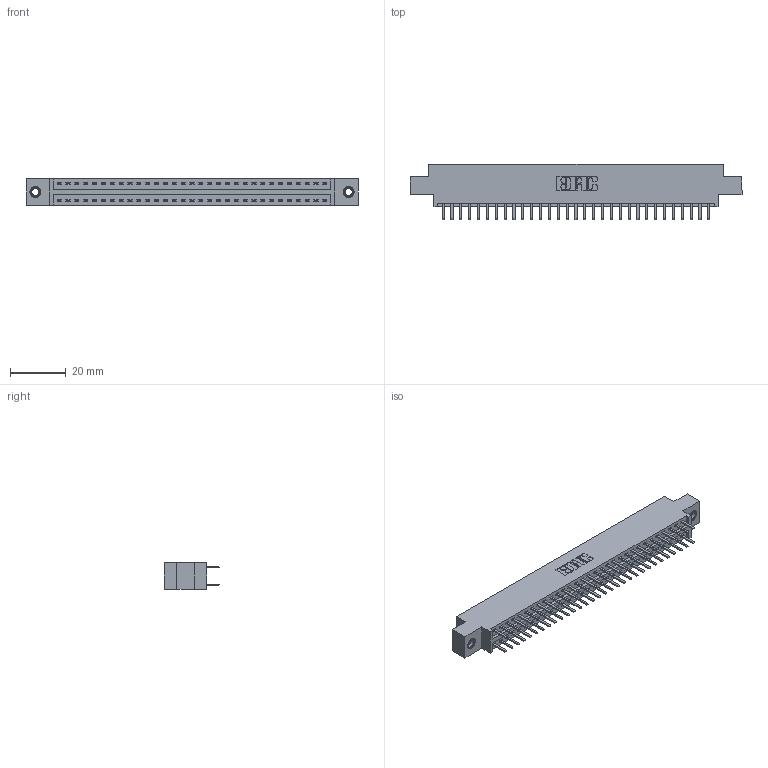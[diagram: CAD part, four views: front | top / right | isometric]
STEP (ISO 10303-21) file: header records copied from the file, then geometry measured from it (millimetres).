
FILE_DESCRIPTION (( 'STEP AP203' ), '1' );
FILE_NAME ('396-062-520-807.STEP', '2019-11-02T09:13:12', ( '' ), ( '' ), 'SwSTEP 2.0', 'SolidWorks 2016', '' );
FILE_SCHEMA (( 'CONFIG_CONTROL_DESIGN' ));
Length unit declared in the file: inch
Products named in the file (4): 346 Part_0.170 Offset - 0.156 Dia-TI; 345-292-001_345-293-120; 345-250-001_345-250-005-103; 396-062-520-807
Assembly tree (65 placements, depth 2):
  396-062-520-807
    346 Part_0.170 Offset - 0.156 Dia-TI
    345-292-001_345-293-120  x62
    345-250-001_345-250-005-103  x2
Bounding box: 119 x 20.02 x 9.4 mm (x, y, z)
Volume: 11323.1 mm3; surface area: 15540.9 mm2
Topology: 65 solids, 65 shells, 3658 faces, 10583 edges, 6882 vertices
Faces by surface type: plane 2406, cylinder 1236, cone 12, torus 4
Entity records: 23144 total; most frequent: CARTESIAN_POINT 3827, ORIENTED_EDGE 3742, DIRECTION 3437, EDGE_CURVE 1871, VECTOR 1591, LINE 1591, VERTEX_POINT 1240, AXIS2_PLACEMENT_3D 923
